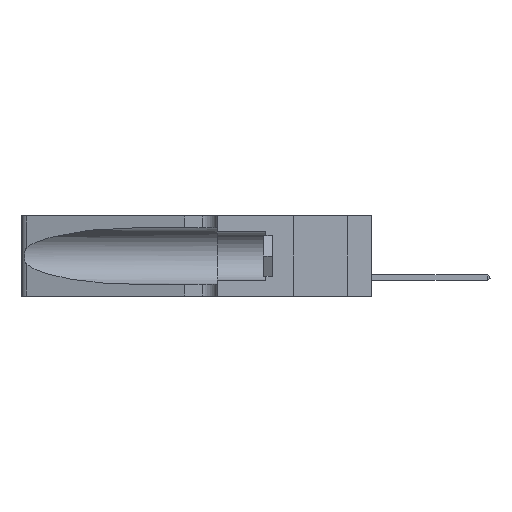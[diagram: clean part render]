
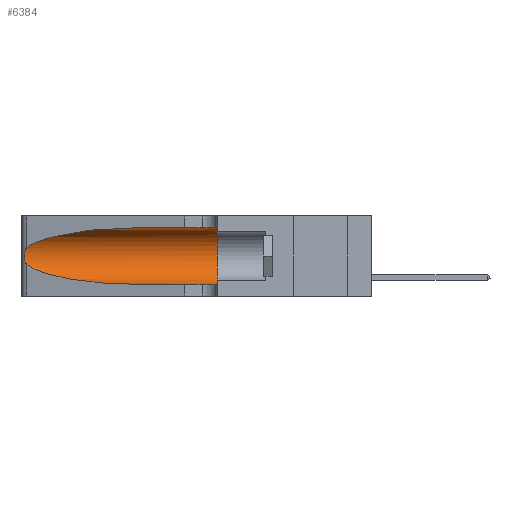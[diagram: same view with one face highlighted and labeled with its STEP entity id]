
A CAD part, left-side view. The second image highlights one B-rep face of the part: STEP entity #6384.
In plain terms, the highlighted cylindrical face has radius 3.308 mm (diameter 6.617 mm), a partial arc.
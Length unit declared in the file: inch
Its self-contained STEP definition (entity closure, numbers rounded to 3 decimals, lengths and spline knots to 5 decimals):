
#239 = CARTESIAN_POINT ( 'NONE',  ( 0.18966, 0.96281, 0.31525 ) ) ;
#828 = CARTESIAN_POINT ( 'NONE',  ( 0.1305, 0.35, 0.185 ) ) ;
#1292 = EDGE_CURVE ( 'NONE', #9347, #2238, #6943, .T. ) ;
#1599 = CARTESIAN_POINT ( 'NONE',  ( 0.26075, 1.23896, 0.178 ) ) ;
#2200 = CARTESIAN_POINT ( 'NONE',  ( 0.1305, 0.35, 0.31525 ) ) ;
#2238 = VERTEX_POINT ( 'NONE', #17943 ) ;
#2327 = EDGE_CURVE ( 'NONE', #11681, #13161, #15576, .T. ) ;
#2581 = VECTOR ( 'NONE', #17911, 39.37008 ) ;
#3140 = DIRECTION ( 'NONE',  ( 0., 0., 1. ) ) ;
#3209 = CARTESIAN_POINT ( 'NONE',  ( 0.25555, 1.22993, 0.14849 ) ) ;
#3450 = CARTESIAN_POINT ( 'NONE',  ( 0.25487, 1.22718, 0.14631 ) ) ;
#3627 = ORIENTED_EDGE ( 'NONE', *, *, #16655, .T. ) ;
#3988 = AXIS2_PLACEMENT_3D ( 'NONE', #828, #17673, #3140 ) ;
#4638 = ORIENTED_EDGE ( 'NONE', *, *, #1292, .T. ) ;
#5814 = CARTESIAN_POINT ( 'NONE',  ( 0.25487, 1.22718, 0.22369 ) ) ;
#6164 = CYLINDRICAL_SURFACE ( 'NONE', #15807, 0.13025 ) ;
#6384 = ADVANCED_FACE ( 'NONE', ( #21394 ), #6164, .F. ) ;
#6943 = B_SPLINE_CURVE_WITH_KNOTS ( 'NONE', 3,
 ( #10811, #23395, #21485, #12635, #8834, #17966, #19705, #1599, #7013, #10569, #12392, #17743, #3209, #3450 ),
 .UNSPECIFIED., .F., .F.,
 ( 4, 2, 2, 2, 2, 2, 4 ),
 ( 0., 0.00027, 0.00053, 0.00107, 0.0016, 0.00187, 0.00214 ),
 .UNSPECIFIED. ) ;
#7013 = CARTESIAN_POINT ( 'NONE',  ( 0.26017, 1.23833, 0.17102 ) ) ;
#8834 = CARTESIAN_POINT ( 'NONE',  ( 0.25854, 1.2359, 0.20912 ) ) ;
#9347 = VERTEX_POINT ( 'NONE', #15995 ) ;
#9531 = CARTESIAN_POINT ( 'NONE',  ( 0.2373, 1.15595, 0.28018 ) ) ;
#10116 = CARTESIAN_POINT ( 'NONE',  ( 0.1305, 1.61858, 0.31525 ) ) ;
#10151 = CARTESIAN_POINT ( 'NONE',  ( 0.1305, 0.35, 0.05475 ) ) ;
#10496 = CIRCLE ( 'NONE', #3988, 0.13025 ) ;
#10569 = CARTESIAN_POINT ( 'NONE',  ( 0.25856, 1.23593, 0.16098 ) ) ;
#10811 = CARTESIAN_POINT ( 'NONE',  ( 0.25487, 1.22718, 0.22369 ) ) ;
#11018 = DIRECTION ( 'NONE',  ( 0., -1., 0. ) ) ;
#11249 = CARTESIAN_POINT ( 'NONE',  ( 0.1305, 1.61858, 0.05475 ) ) ;
#11336 = EDGE_CURVE ( 'NONE', #13504, #21980, #20120, .T. ) ;
#11681 = VERTEX_POINT ( 'NONE', #18621 ) ;
#12392 = CARTESIAN_POINT ( 'NONE',  ( 0.25789, 1.23486, 0.15765 ) ) ;
#12470 = ORIENTED_EDGE ( 'NONE', *, *, #17407, .T. ) ;
#12635 = CARTESIAN_POINT ( 'NONE',  ( 0.25787, 1.23484, 0.2124 ) ) ;
#12657 = CARTESIAN_POINT ( 'NONE',  ( 0.25487, 1.22718, 0.14631 ) ) ;
#13161 = VERTEX_POINT ( 'NONE', #10151 ) ;
#13466 =( BOUNDED_CURVE ( )  B_SPLINE_CURVE ( 3, ( #18266, #239, #9531, #5814 ),
 .UNSPECIFIED., .F., .T. ) 
 B_SPLINE_CURVE_WITH_KNOTS ( ( 4, 4 ),
 ( 1.5708, 2.84003 ),
 .UNSPECIFIED. ) 
 CURVE ( )  GEOMETRIC_REPRESENTATION_ITEM ( )  RATIONAL_B_SPLINE_CURVE ( ( 1., 0.87, 0.87, 1. ) ) 
 REPRESENTATION_ITEM ( '' )  );
#13504 = VERTEX_POINT ( 'NONE', #20109 ) ;
#14869 = DIRECTION ( 'NONE',  ( 0., 0., -1. ) ) ;
#15576 = LINE ( 'NONE', #11249, #19221 ) ;
#15807 = AXIS2_PLACEMENT_3D ( 'NONE', #18562, #22308, #14869 ) ;
#15995 = CARTESIAN_POINT ( 'NONE',  ( 0.25487, 1.22718, 0.22369 ) ) ;
#16345 = CARTESIAN_POINT ( 'NONE',  ( 0.2373, 1.15595, 0.08982 ) ) ;
#16655 = EDGE_CURVE ( 'NONE', #2238, #11681, #22371, .T. ) ;
#16969 = ORIENTED_EDGE ( 'NONE', *, *, #22505, .F. ) ;
#17407 = EDGE_CURVE ( 'NONE', #13504, #9347, #13466, .T. ) ;
#17673 = DIRECTION ( 'NONE',  ( 0., 1., 0. ) ) ;
#17743 = CARTESIAN_POINT ( 'NONE',  ( 0.25639, 1.23186, 0.15144 ) ) ;
#17911 = DIRECTION ( 'NONE',  ( 0., -1., 0. ) ) ;
#17943 = CARTESIAN_POINT ( 'NONE',  ( 0.25487, 1.22718, 0.14631 ) ) ;
#17966 = CARTESIAN_POINT ( 'NONE',  ( 0.26018, 1.23835, 0.19895 ) ) ;
#18266 = CARTESIAN_POINT ( 'NONE',  ( 0.1305, 0.72297, 0.31525 ) ) ;
#18562 = CARTESIAN_POINT ( 'NONE',  ( 0.1305, 1.61858, 0.185 ) ) ;
#18621 = CARTESIAN_POINT ( 'NONE',  ( 0.1305, 0.72297, 0.05475 ) ) ;
#19197 = ORIENTED_EDGE ( 'NONE', *, *, #2327, .T. ) ;
#19221 = VECTOR ( 'NONE', #11018, 39.37008 ) ;
#19705 = CARTESIAN_POINT ( 'NONE',  ( 0.26075, 1.23896, 0.19203 ) ) ;
#19957 = ORIENTED_EDGE ( 'NONE', *, *, #11336, .F. ) ;
#20045 = CARTESIAN_POINT ( 'NONE',  ( 0.18966, 0.96281, 0.05475 ) ) ;
#20109 = CARTESIAN_POINT ( 'NONE',  ( 0.1305, 0.72297, 0.31525 ) ) ;
#20120 = LINE ( 'NONE', #10116, #2581 ) ;
#21394 = FACE_OUTER_BOUND ( 'NONE', #21901, .T. ) ;
#21485 = CARTESIAN_POINT ( 'NONE',  ( 0.25639, 1.23184, 0.21858 ) ) ;
#21901 = EDGE_LOOP ( 'NONE', ( #12470, #4638, #3627, #19197, #16969, #19957 ) ) ;
#21980 = VERTEX_POINT ( 'NONE', #2200 ) ;
#22308 = DIRECTION ( 'NONE',  ( 0., -1., 0. ) ) ;
#22371 =( BOUNDED_CURVE ( )  B_SPLINE_CURVE ( 3, ( #12657, #16345, #20045, #23336 ),
 .UNSPECIFIED., .F., .F. ) 
 B_SPLINE_CURVE_WITH_KNOTS ( ( 4, 4 ),
 ( 3.44316, 4.71239 ),
 .UNSPECIFIED. ) 
 CURVE ( )  GEOMETRIC_REPRESENTATION_ITEM ( )  RATIONAL_B_SPLINE_CURVE ( ( 1., 0.87, 0.87, 1. ) ) 
 REPRESENTATION_ITEM ( '' )  );
#22505 = EDGE_CURVE ( 'NONE', #21980, #13161, #10496, .T. ) ;
#23336 = CARTESIAN_POINT ( 'NONE',  ( 0.1305, 0.72297, 0.05475 ) ) ;
#23395 = CARTESIAN_POINT ( 'NONE',  ( 0.25555, 1.22994, 0.2215 ) ) ;
